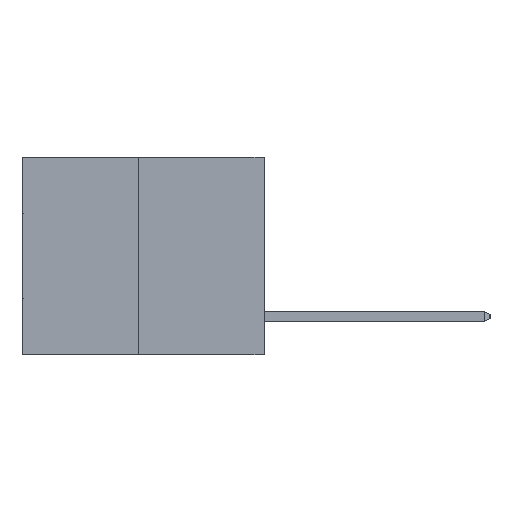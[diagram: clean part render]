
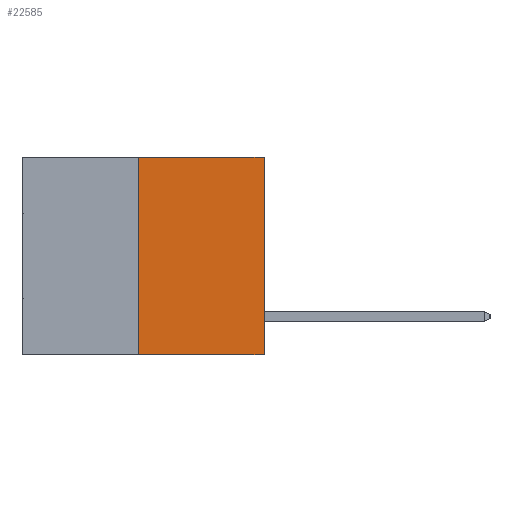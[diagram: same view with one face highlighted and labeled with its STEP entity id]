
A CAD part, left-side view. The second image highlights one B-rep face of the part: STEP entity #22585.
In plain terms, the highlighted planar face has unit normal (-1, 0, 0).
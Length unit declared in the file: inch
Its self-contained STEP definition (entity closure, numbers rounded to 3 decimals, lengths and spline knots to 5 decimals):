
#1315 = CARTESIAN_POINT ( 'NONE',  ( 0., 0.312, -0.49 ) ) ;
#1428 = VERTEX_POINT ( 'NONE', #14565 ) ;
#1675 = DIRECTION ( 'NONE',  ( 0., -1., 0. ) ) ;
#2542 = DIRECTION ( 'NONE',  ( 0., 0., 1. ) ) ;
#2778 = VECTOR ( 'NONE', #23962, 39.37008 ) ;
#2792 = EDGE_LOOP ( 'NONE', ( #21826, #15845, #31423, #5047 ) ) ;
#3681 = AXIS2_PLACEMENT_3D ( 'NONE', #30273, #25306, #12860 ) ;
#4671 = LINE ( 'NONE', #30244, #6241 ) ;
#5047 = ORIENTED_EDGE ( 'NONE', *, *, #31988, .F. ) ;
#5754 = VECTOR ( 'NONE', #1675, 39.37008 ) ;
#6241 = VECTOR ( 'NONE', #2542, 39.37008 ) ;
#6601 = VERTEX_POINT ( 'NONE', #1315 ) ;
#8230 = LINE ( 'NONE', #8345, #29125 ) ;
#8345 = CARTESIAN_POINT ( 'NONE',  ( 0., 0.6, 0. ) ) ;
#12860 = DIRECTION ( 'NONE',  ( 0., 0., -1. ) ) ;
#12893 = EDGE_CURVE ( 'NONE', #28704, #1428, #19664, .T. ) ;
#14209 = CARTESIAN_POINT ( 'NONE',  ( 0., 0.6, -0.49 ) ) ;
#14565 = CARTESIAN_POINT ( 'NONE',  ( 0., 0., 0. ) ) ;
#15478 = CARTESIAN_POINT ( 'NONE',  ( 0., 0.312, 0. ) ) ;
#15845 = ORIENTED_EDGE ( 'NONE', *, *, #26403, .T. ) ;
#19664 = LINE ( 'NONE', #31894, #2778 ) ;
#20175 = EDGE_CURVE ( 'NONE', #6601, #27508, #4671, .T. ) ;
#20428 = CARTESIAN_POINT ( 'NONE',  ( 0., 0., -0.49 ) ) ;
#20717 = PLANE ( 'NONE',  #3681 ) ;
#21826 = ORIENTED_EDGE ( 'NONE', *, *, #20175, .F. ) ;
#22585 = ADVANCED_FACE ( 'NONE', ( #28142 ), #20717, .F. ) ;
#23962 = DIRECTION ( 'NONE',  ( 0., 0., 1. ) ) ;
#25306 = DIRECTION ( 'NONE',  ( 1., 0., 0. ) ) ;
#26403 = EDGE_CURVE ( 'NONE', #6601, #28704, #26580, .T. ) ;
#26580 = LINE ( 'NONE', #14209, #5754 ) ;
#27508 = VERTEX_POINT ( 'NONE', #15478 ) ;
#28142 = FACE_OUTER_BOUND ( 'NONE', #2792, .T. ) ;
#28704 = VERTEX_POINT ( 'NONE', #20428 ) ;
#29125 = VECTOR ( 'NONE', #31027, 39.37008 ) ;
#30244 = CARTESIAN_POINT ( 'NONE',  ( 0., 0.312, -0.49 ) ) ;
#30273 = CARTESIAN_POINT ( 'NONE',  ( 0., 0.6, 0. ) ) ;
#31027 = DIRECTION ( 'NONE',  ( 0., -1., 0. ) ) ;
#31423 = ORIENTED_EDGE ( 'NONE', *, *, #12893, .T. ) ;
#31894 = CARTESIAN_POINT ( 'NONE',  ( 0., 0., 0. ) ) ;
#31988 = EDGE_CURVE ( 'NONE', #27508, #1428, #8230, .T. ) ;
